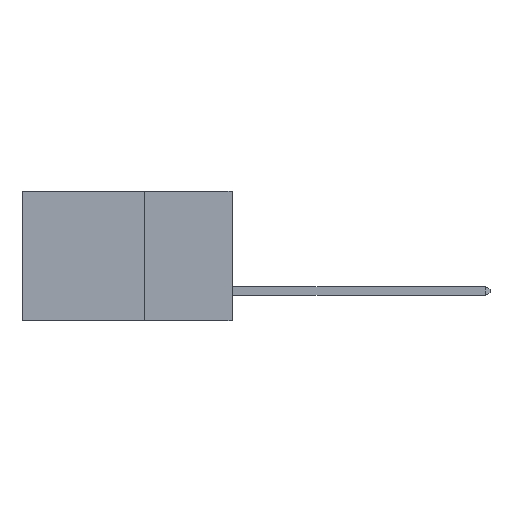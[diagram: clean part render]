
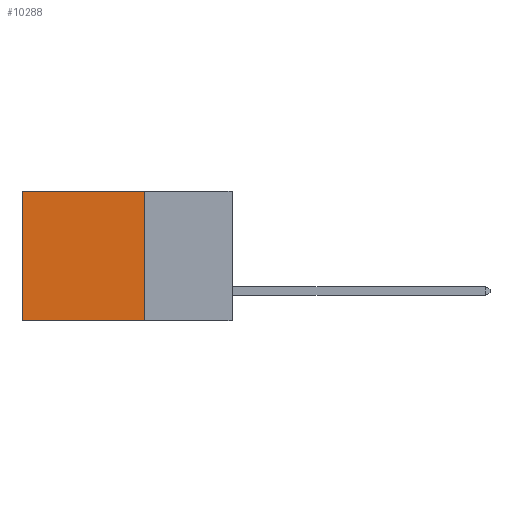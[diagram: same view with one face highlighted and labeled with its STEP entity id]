
A CAD part, left-side view. The second image highlights one B-rep face of the part: STEP entity #10288.
In plain terms, the highlighted planar face has unit normal (-1, 0, 0).
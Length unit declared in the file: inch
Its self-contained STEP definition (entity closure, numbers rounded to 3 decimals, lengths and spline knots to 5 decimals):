
#338 = CARTESIAN_POINT ( 'NONE',  ( 0.2875, 0.25, 0. ) ) ;
#595 = LINE ( 'NONE', #1514, #5545 ) ;
#786 = ORIENTED_EDGE ( 'NONE', *, *, #4040, .T. ) ;
#1156 = ORIENTED_EDGE ( 'NONE', *, *, #7913, .F. ) ;
#1484 = VECTOR ( 'NONE', #1963, 39.37008 ) ;
#1514 = CARTESIAN_POINT ( 'NONE',  ( 0.2875, 0.25, -0.37 ) ) ;
#1963 = DIRECTION ( 'NONE',  ( 0., 1., 0. ) ) ;
#2029 = ORIENTED_EDGE ( 'NONE', *, *, #4142, .F. ) ;
#2077 = AXIS2_PLACEMENT_3D ( 'NONE', #9845, #4270, #10801 ) ;
#2216 = VERTEX_POINT ( 'NONE', #10894 ) ;
#2306 = VERTEX_POINT ( 'NONE', #10108 ) ;
#4040 = EDGE_CURVE ( 'NONE', #7055, #2306, #4147, .T. ) ;
#4104 = ORIENTED_EDGE ( 'NONE', *, *, #9953, .T. ) ;
#4142 = EDGE_CURVE ( 'NONE', #2216, #11531, #595, .T. ) ;
#4147 = LINE ( 'NONE', #338, #1484 ) ;
#4202 = VECTOR ( 'NONE', #6481, 39.37008 ) ;
#4270 = DIRECTION ( 'NONE',  ( 1., 0., 0. ) ) ;
#5545 = VECTOR ( 'NONE', #9230, 39.37008 ) ;
#5757 = FACE_OUTER_BOUND ( 'NONE', #8145, .T. ) ;
#6481 = DIRECTION ( 'NONE',  ( 0., 0., -1. ) ) ;
#6829 = CARTESIAN_POINT ( 'NONE',  ( 0.2875, 0.25, 0. ) ) ;
#7055 = VERTEX_POINT ( 'NONE', #6829 ) ;
#7913 = EDGE_CURVE ( 'NONE', #7055, #2216, #8844, .T. ) ;
#8145 = EDGE_LOOP ( 'NONE', ( #4104, #2029, #1156, #786 ) ) ;
#8844 = LINE ( 'NONE', #8962, #10985 ) ;
#8962 = CARTESIAN_POINT ( 'NONE',  ( 0.2875, 0.25, 0. ) ) ;
#9230 = DIRECTION ( 'NONE',  ( 0., 1., 0. ) ) ;
#9845 = CARTESIAN_POINT ( 'NONE',  ( 0.2875, 0.25, 0. ) ) ;
#9872 = DIRECTION ( 'NONE',  ( 0., 0., -1. ) ) ;
#9886 = PLANE ( 'NONE',  #2077 ) ;
#9953 = EDGE_CURVE ( 'NONE', #2306, #11531, #11615, .T. ) ;
#10108 = CARTESIAN_POINT ( 'NONE',  ( 0.2875, 0.6, 0. ) ) ;
#10117 = CARTESIAN_POINT ( 'NONE',  ( 0.2875, 0.6, 0. ) ) ;
#10288 = ADVANCED_FACE ( 'NONE', ( #5757 ), #9886, .F. ) ;
#10736 = CARTESIAN_POINT ( 'NONE',  ( 0.2875, 0.6, -0.37 ) ) ;
#10801 = DIRECTION ( 'NONE',  ( 0., 0., -1. ) ) ;
#10894 = CARTESIAN_POINT ( 'NONE',  ( 0.2875, 0.25, -0.37 ) ) ;
#10985 = VECTOR ( 'NONE', #9872, 39.37008 ) ;
#11531 = VERTEX_POINT ( 'NONE', #10736 ) ;
#11615 = LINE ( 'NONE', #10117, #4202 ) ;
